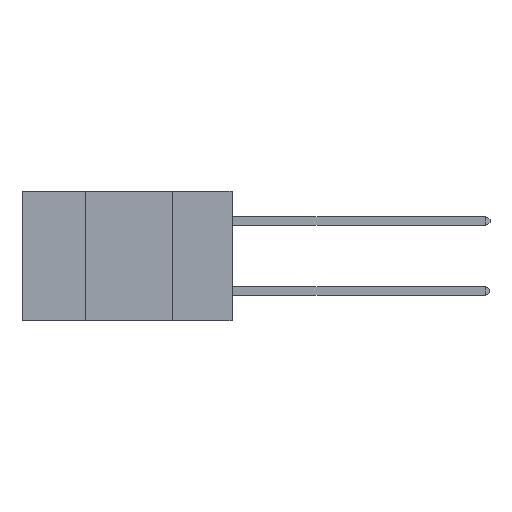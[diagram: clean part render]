
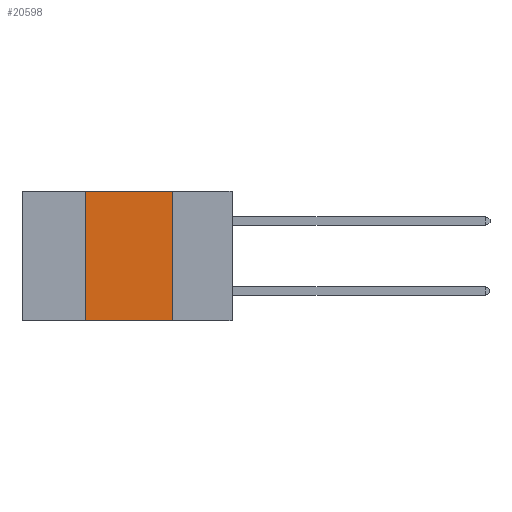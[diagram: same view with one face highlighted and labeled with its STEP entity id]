
A CAD part, left-side view. The second image highlights one B-rep face of the part: STEP entity #20598.
In plain terms, the highlighted planar face has unit normal (-1, 0, 0).
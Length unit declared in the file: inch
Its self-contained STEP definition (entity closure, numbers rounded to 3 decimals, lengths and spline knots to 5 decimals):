
#507 = CARTESIAN_POINT ( 'NONE',  ( 0., 0.42, -0.37 ) ) ;
#1312 = EDGE_CURVE ( 'NONE', #18301, #15388, #6737, .T. ) ;
#1671 = CARTESIAN_POINT ( 'NONE',  ( 0., 0.17, 0. ) ) ;
#2622 = VERTEX_POINT ( 'NONE', #507 ) ;
#3928 = ORIENTED_EDGE ( 'NONE', *, *, #13195, .F. ) ;
#4058 = CARTESIAN_POINT ( 'NONE',  ( 0., 0.17, -0.37 ) ) ;
#5266 = CARTESIAN_POINT ( 'NONE',  ( 0., 0.6, 0. ) ) ;
#5444 = LINE ( 'NONE', #19709, #13628 ) ;
#6737 = LINE ( 'NONE', #8562, #10510 ) ;
#6911 = DIRECTION ( 'NONE',  ( 0., 0., -1. ) ) ;
#8101 = ORIENTED_EDGE ( 'NONE', *, *, #1312, .F. ) ;
#8125 = CARTESIAN_POINT ( 'NONE',  ( 0., 0.6, -0.37 ) ) ;
#8562 = CARTESIAN_POINT ( 'NONE',  ( 0., 0.6, 0. ) ) ;
#8909 = VECTOR ( 'NONE', #9499, 39.37008 ) ;
#9456 = VERTEX_POINT ( 'NONE', #4058 ) ;
#9499 = DIRECTION ( 'NONE',  ( 0., 0., -1. ) ) ;
#9855 = EDGE_CURVE ( 'NONE', #2622, #9456, #20660, .T. ) ;
#10510 = VECTOR ( 'NONE', #12108, 39.37008 ) ;
#10767 = EDGE_LOOP ( 'NONE', ( #16458, #8101, #3928, #15956 ) ) ;
#11070 = CARTESIAN_POINT ( 'NONE',  ( 0., 0.17, 0. ) ) ;
#11910 = VECTOR ( 'NONE', #18157, 39.37008 ) ;
#12108 = DIRECTION ( 'NONE',  ( 0., -1., 0. ) ) ;
#13195 = EDGE_CURVE ( 'NONE', #2622, #18301, #5444, .T. ) ;
#13628 = VECTOR ( 'NONE', #21294, 39.37008 ) ;
#13936 = AXIS2_PLACEMENT_3D ( 'NONE', #5266, #16736, #6911 ) ;
#14304 = EDGE_CURVE ( 'NONE', #15388, #9456, #18238, .T. ) ;
#15388 = VERTEX_POINT ( 'NONE', #1671 ) ;
#15956 = ORIENTED_EDGE ( 'NONE', *, *, #9855, .T. ) ;
#16458 = ORIENTED_EDGE ( 'NONE', *, *, #14304, .F. ) ;
#16736 = DIRECTION ( 'NONE',  ( 1., 0., 0. ) ) ;
#18157 = DIRECTION ( 'NONE',  ( 0., -1., 0. ) ) ;
#18238 = LINE ( 'NONE', #11070, #8909 ) ;
#18301 = VERTEX_POINT ( 'NONE', #19321 ) ;
#19321 = CARTESIAN_POINT ( 'NONE',  ( 0., 0.42, 0. ) ) ;
#19709 = CARTESIAN_POINT ( 'NONE',  ( 0., 0.42, 0. ) ) ;
#19783 = FACE_OUTER_BOUND ( 'NONE', #10767, .T. ) ;
#19943 = PLANE ( 'NONE',  #13936 ) ;
#20598 = ADVANCED_FACE ( 'NONE', ( #19783 ), #19943, .F. ) ;
#20660 = LINE ( 'NONE', #8125, #11910 ) ;
#21294 = DIRECTION ( 'NONE',  ( 0., 0., 1. ) ) ;
